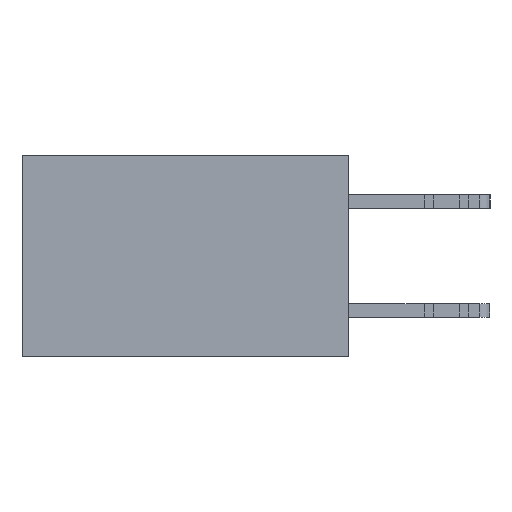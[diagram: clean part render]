
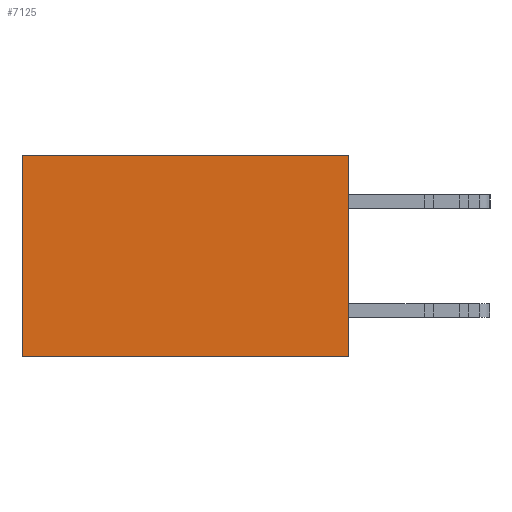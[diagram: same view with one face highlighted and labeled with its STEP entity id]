
A CAD part, left-side view. The second image highlights one B-rep face of the part: STEP entity #7125.
In plain terms, the highlighted planar face has unit normal (-1, 0, 0).
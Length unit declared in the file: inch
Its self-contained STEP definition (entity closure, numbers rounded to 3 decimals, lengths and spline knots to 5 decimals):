
#151 = CARTESIAN_POINT ( 'NONE',  ( 0.2615, 0., -0.37 ) ) ;
#549 = FACE_OUTER_BOUND ( 'NONE', #12888, .T. ) ;
#669 = DIRECTION ( 'NONE',  ( 0., 0., -1. ) ) ;
#1223 = ORIENTED_EDGE ( 'NONE', *, *, #9242, .T. ) ;
#1689 = CARTESIAN_POINT ( 'NONE',  ( 0.2615, 0., -0.37 ) ) ;
#2902 = ORIENTED_EDGE ( 'NONE', *, *, #16139, .T. ) ;
#3420 = CARTESIAN_POINT ( 'NONE',  ( 0.2615, 0., 0. ) ) ;
#3492 = CARTESIAN_POINT ( 'NONE',  ( 0.2615, 0.6, -0.37 ) ) ;
#3767 = VERTEX_POINT ( 'NONE', #1689 ) ;
#4124 = VERTEX_POINT ( 'NONE', #3420 ) ;
#4314 = CARTESIAN_POINT ( 'NONE',  ( 0.2615, 0., -0.37 ) ) ;
#4499 = VECTOR ( 'NONE', #23945, 39.37008 ) ;
#5133 = DIRECTION ( 'NONE',  ( 0., 0., -1. ) ) ;
#5281 = ORIENTED_EDGE ( 'NONE', *, *, #7513, .F. ) ;
#7125 = ADVANCED_FACE ( 'NONE', ( #549 ), #8206, .F. ) ;
#7513 = EDGE_CURVE ( 'NONE', #3767, #14799, #21111, .T. ) ;
#8206 = PLANE ( 'NONE',  #8299 ) ;
#8299 = AXIS2_PLACEMENT_3D ( 'NONE', #4314, #19373, #669 ) ;
#9242 = EDGE_CURVE ( 'NONE', #4124, #22178, #12480, .T. ) ;
#10108 = DIRECTION ( 'NONE',  ( 0., 0., -1. ) ) ;
#10747 = CARTESIAN_POINT ( 'NONE',  ( 0.2615, 0., 0. ) ) ;
#11981 = CARTESIAN_POINT ( 'NONE',  ( 0.2615, 0.6, 0. ) ) ;
#12135 = EDGE_CURVE ( 'NONE', #4124, #3767, #14443, .T. ) ;
#12480 = LINE ( 'NONE', #10747, #4499 ) ;
#12888 = EDGE_LOOP ( 'NONE', ( #2902, #5281, #22166, #1223 ) ) ;
#14443 = LINE ( 'NONE', #22031, #15829 ) ;
#14799 = VERTEX_POINT ( 'NONE', #3492 ) ;
#15085 = LINE ( 'NONE', #20181, #19845 ) ;
#15829 = VECTOR ( 'NONE', #10108, 39.37008 ) ;
#16139 = EDGE_CURVE ( 'NONE', #22178, #14799, #15085, .T. ) ;
#18591 = VECTOR ( 'NONE', #22864, 39.37008 ) ;
#19373 = DIRECTION ( 'NONE',  ( 1., 0., 0. ) ) ;
#19845 = VECTOR ( 'NONE', #5133, 39.37008 ) ;
#20181 = CARTESIAN_POINT ( 'NONE',  ( 0.2615, 0.6, -0.37 ) ) ;
#21111 = LINE ( 'NONE', #151, #18591 ) ;
#22031 = CARTESIAN_POINT ( 'NONE',  ( 0.2615, 0., -0.37 ) ) ;
#22166 = ORIENTED_EDGE ( 'NONE', *, *, #12135, .F. ) ;
#22178 = VERTEX_POINT ( 'NONE', #11981 ) ;
#22864 = DIRECTION ( 'NONE',  ( 0., 1., 0. ) ) ;
#23945 = DIRECTION ( 'NONE',  ( 0., 1., 0. ) ) ;
